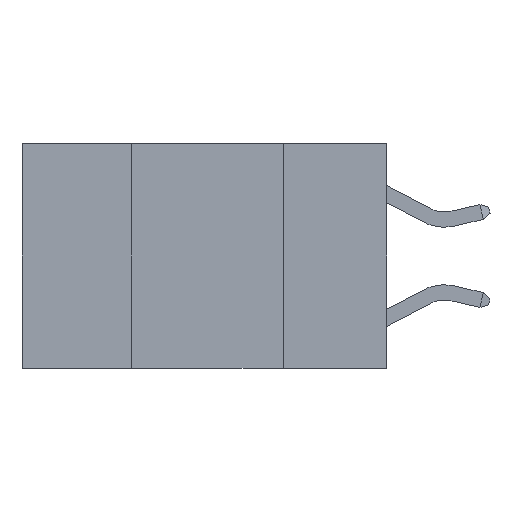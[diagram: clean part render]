
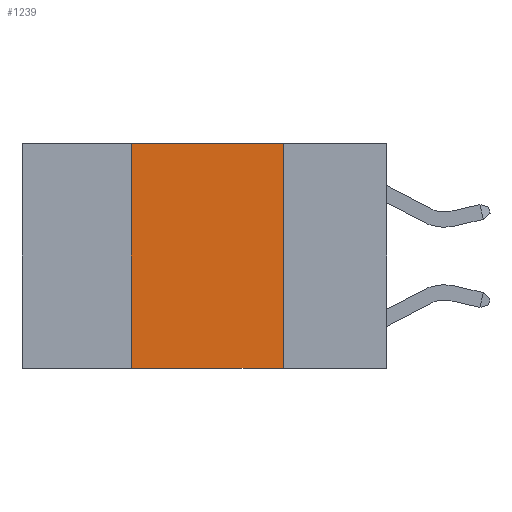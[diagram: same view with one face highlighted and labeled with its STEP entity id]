
A CAD part, left-side view. The second image highlights one B-rep face of the part: STEP entity #1239.
In plain terms, the highlighted planar face has unit normal (-1, 0, 0).
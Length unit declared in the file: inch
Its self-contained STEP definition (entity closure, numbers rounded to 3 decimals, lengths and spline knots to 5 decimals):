
#152 = LINE ( 'NONE', #15733, #12980 ) ;
#977 = DIRECTION ( 'NONE',  ( 0., 0., 1. ) ) ;
#1065 = ORIENTED_EDGE ( 'NONE', *, *, #10604, .F. ) ;
#1239 = ADVANCED_FACE ( 'NONE', ( #7444 ), #16011, .F. ) ;
#1529 = EDGE_LOOP ( 'NONE', ( #8255, #6318, #1065, #7522 ) ) ;
#1766 = VERTEX_POINT ( 'NONE', #3782 ) ;
#1876 = DIRECTION ( 'NONE',  ( 0., -1., 0. ) ) ;
#2494 = CARTESIAN_POINT ( 'NONE',  ( 0., 0.17, 0. ) ) ;
#2803 = EDGE_CURVE ( 'NONE', #10599, #11240, #7203, .T. ) ;
#3782 = CARTESIAN_POINT ( 'NONE',  ( 0., 0.17, -0.37 ) ) ;
#6181 = CARTESIAN_POINT ( 'NONE',  ( 0., 0.42, 0. ) ) ;
#6318 = ORIENTED_EDGE ( 'NONE', *, *, #2803, .F. ) ;
#6864 = LINE ( 'NONE', #7439, #9878 ) ;
#6888 = VERTEX_POINT ( 'NONE', #9568 ) ;
#7203 = LINE ( 'NONE', #9615, #11006 ) ;
#7439 = CARTESIAN_POINT ( 'NONE',  ( 0., 0.42, 0. ) ) ;
#7444 = FACE_OUTER_BOUND ( 'NONE', #1529, .T. ) ;
#7522 = ORIENTED_EDGE ( 'NONE', *, *, #9775, .T. ) ;
#8255 = ORIENTED_EDGE ( 'NONE', *, *, #12265, .F. ) ;
#8321 = DIRECTION ( 'NONE',  ( 0., -1., 0. ) ) ;
#8615 = DIRECTION ( 'NONE',  ( 0., 0., -1. ) ) ;
#9568 = CARTESIAN_POINT ( 'NONE',  ( 0., 0.42, -0.37 ) ) ;
#9615 = CARTESIAN_POINT ( 'NONE',  ( 0., 0.6, 0. ) ) ;
#9775 = EDGE_CURVE ( 'NONE', #6888, #1766, #152, .T. ) ;
#9878 = VECTOR ( 'NONE', #977, 39.37008 ) ;
#10026 = AXIS2_PLACEMENT_3D ( 'NONE', #15784, #15734, #15731 ) ;
#10599 = VERTEX_POINT ( 'NONE', #6181 ) ;
#10604 = EDGE_CURVE ( 'NONE', #6888, #10599, #6864, .T. ) ;
#11006 = VECTOR ( 'NONE', #1876, 39.37008 ) ;
#11240 = VERTEX_POINT ( 'NONE', #2494 ) ;
#12265 = EDGE_CURVE ( 'NONE', #11240, #1766, #15669, .T. ) ;
#12431 = VECTOR ( 'NONE', #8615, 39.37008 ) ;
#12980 = VECTOR ( 'NONE', #8321, 39.37008 ) ;
#13553 = CARTESIAN_POINT ( 'NONE',  ( 0., 0.17, 0. ) ) ;
#15669 = LINE ( 'NONE', #13553, #12431 ) ;
#15731 = DIRECTION ( 'NONE',  ( 0., 0., -1. ) ) ;
#15733 = CARTESIAN_POINT ( 'NONE',  ( 0., 0.6, -0.37 ) ) ;
#15734 = DIRECTION ( 'NONE',  ( 1., 0., 0. ) ) ;
#15784 = CARTESIAN_POINT ( 'NONE',  ( 0., 0.6, 0. ) ) ;
#16011 = PLANE ( 'NONE',  #10026 ) ;
